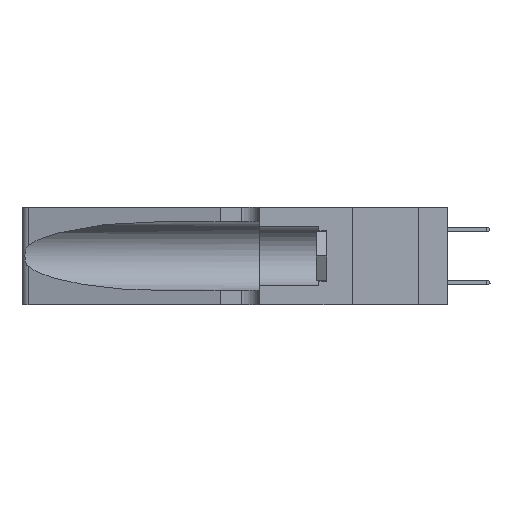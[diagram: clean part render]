
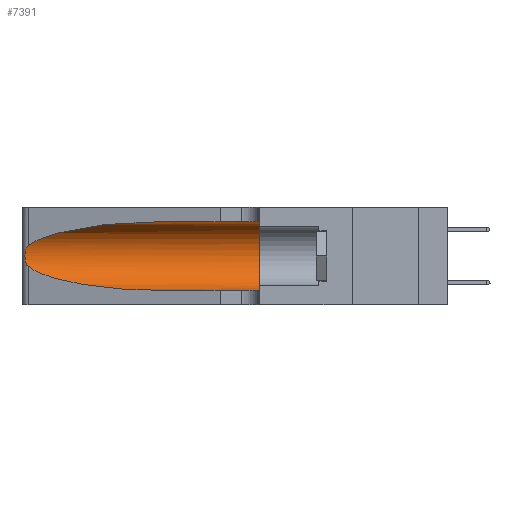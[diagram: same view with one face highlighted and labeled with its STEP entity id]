
A CAD part, left-side view. The second image highlights one B-rep face of the part: STEP entity #7391.
In plain terms, the highlighted cylindrical face has radius 3.308 mm (diameter 6.617 mm), a partial arc.
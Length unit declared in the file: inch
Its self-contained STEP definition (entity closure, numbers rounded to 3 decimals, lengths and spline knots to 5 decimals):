
#606 = CARTESIAN_POINT ( 'NONE',  ( 0.26017, 1.23833, 0.17102 ) ) ;
#2856 = EDGE_CURVE ( 'NONE', #10969, #3639, #28377, .T. ) ;
#3639 = VERTEX_POINT ( 'NONE', #48839 ) ;
#4372 = CARTESIAN_POINT ( 'NONE',  ( 0.25487, 1.22718, 0.22369 ) ) ;
#4533 = CARTESIAN_POINT ( 'NONE',  ( 0.25789, 1.23486, 0.15765 ) ) ;
#5224 = DIRECTION ( 'NONE',  ( 0., -1., 0. ) ) ;
#5656 = CARTESIAN_POINT ( 'NONE',  ( 0.1305, 1.61858, 0.05475 ) ) ;
#5905 = EDGE_CURVE ( 'NONE', #47473, #48548, #41609, .T. ) ;
#6003 = CARTESIAN_POINT ( 'NONE',  ( 0.25487, 1.22718, 0.14631 ) ) ;
#6124 = ORIENTED_EDGE ( 'NONE', *, *, #35734, .F. ) ;
#7391 = ADVANCED_FACE ( 'NONE', ( #47871 ), #16689, .F. ) ;
#8394 = CARTESIAN_POINT ( 'NONE',  ( 0.25555, 1.22993, 0.14849 ) ) ;
#8513 = EDGE_CURVE ( 'NONE', #26982, #40452, #19558, .T. ) ;
#10969 = VERTEX_POINT ( 'NONE', #30127 ) ;
#11135 = CARTESIAN_POINT ( 'NONE',  ( 0.2373, 1.15595, 0.08982 ) ) ;
#11461 = CARTESIAN_POINT ( 'NONE',  ( 0.18966, 0.96281, 0.05475 ) ) ;
#14625 = LINE ( 'NONE', #5656, #23511 ) ;
#15844 = CARTESIAN_POINT ( 'NONE',  ( 0.25787, 1.23484, 0.2124 ) ) ;
#16093 = ORIENTED_EDGE ( 'NONE', *, *, #2856, .T. ) ;
#16689 = CYLINDRICAL_SURFACE ( 'NONE', #29745, 0.13025 ) ;
#19558 =( BOUNDED_CURVE ( )  B_SPLINE_CURVE ( 3, ( #30328, #11135, #11461, #37866 ),
 .UNSPECIFIED., .F., .F. ) 
 B_SPLINE_CURVE_WITH_KNOTS ( ( 4, 4 ),
 ( 3.44316, 4.71239 ),
 .UNSPECIFIED. ) 
 CURVE ( )  GEOMETRIC_REPRESENTATION_ITEM ( )  RATIONAL_B_SPLINE_CURVE ( ( 1., 0.87, 0.87, 1. ) ) 
 REPRESENTATION_ITEM ( '' )  );
#19678 = CARTESIAN_POINT ( 'NONE',  ( 0.26018, 1.23835, 0.19895 ) ) ;
#20430 = CARTESIAN_POINT ( 'NONE',  ( 0.1305, 0.35, 0.185 ) ) ;
#22636 = CARTESIAN_POINT ( 'NONE',  ( 0.1305, 1.61858, 0.31525 ) ) ;
#23462 = CARTESIAN_POINT ( 'NONE',  ( 0.26075, 1.23896, 0.178 ) ) ;
#23511 = VECTOR ( 'NONE', #35915, 39.37008 ) ;
#24247 = DIRECTION ( 'NONE',  ( 0., 0., 1. ) ) ;
#24736 = B_SPLINE_CURVE_WITH_KNOTS ( 'NONE', 3,
 ( #4372, #42047, #38439, #15844, #42210, #19678, #45951, #23462, #606, #27323, #4533, #31049, #8394, #34835 ),
 .UNSPECIFIED., .F., .F.,
 ( 4, 2, 2, 2, 2, 2, 4 ),
 ( 0., 0.00027, 0.00053, 0.00107, 0.0016, 0.00187, 0.00214 ),
 .UNSPECIFIED. ) ;
#26568 = CARTESIAN_POINT ( 'NONE',  ( 0.18966, 0.96281, 0.31525 ) ) ;
#26982 = VERTEX_POINT ( 'NONE', #6003 ) ;
#27323 = CARTESIAN_POINT ( 'NONE',  ( 0.25856, 1.23593, 0.16098 ) ) ;
#27991 = CARTESIAN_POINT ( 'NONE',  ( 0.1305, 1.61858, 0.185 ) ) ;
#28377 =( BOUNDED_CURVE ( )  B_SPLINE_CURVE ( 3, ( #30321, #26568, #48971, #34089 ),
 .UNSPECIFIED., .F., .F. ) 
 B_SPLINE_CURVE_WITH_KNOTS ( ( 4, 4 ),
 ( 1.5708, 2.84003 ),
 .UNSPECIFIED. ) 
 CURVE ( )  GEOMETRIC_REPRESENTATION_ITEM ( )  RATIONAL_B_SPLINE_CURVE ( ( 1., 0.87, 0.87, 1. ) ) 
 REPRESENTATION_ITEM ( '' )  );
#29745 = AXIS2_PLACEMENT_3D ( 'NONE', #27991, #5224, #31721 ) ;
#30127 = CARTESIAN_POINT ( 'NONE',  ( 0.1305, 0.72297, 0.31525 ) ) ;
#30321 = CARTESIAN_POINT ( 'NONE',  ( 0.1305, 0.72297, 0.31525 ) ) ;
#30328 = CARTESIAN_POINT ( 'NONE',  ( 0.25487, 1.22718, 0.14631 ) ) ;
#30532 = CARTESIAN_POINT ( 'NONE',  ( 0.1305, 0.72297, 0.05475 ) ) ;
#30937 = AXIS2_PLACEMENT_3D ( 'NONE', #20430, #46700, #24247 ) ;
#31049 = CARTESIAN_POINT ( 'NONE',  ( 0.25639, 1.23186, 0.15144 ) ) ;
#31544 = ORIENTED_EDGE ( 'NONE', *, *, #5905, .F. ) ;
#31620 = EDGE_CURVE ( 'NONE', #3639, #26982, #24736, .T. ) ;
#31721 = DIRECTION ( 'NONE',  ( 0., 0., -1. ) ) ;
#32508 = EDGE_CURVE ( 'NONE', #40452, #48548, #14625, .T. ) ;
#34089 = CARTESIAN_POINT ( 'NONE',  ( 0.25487, 1.22718, 0.22369 ) ) ;
#34835 = CARTESIAN_POINT ( 'NONE',  ( 0.25487, 1.22718, 0.14631 ) ) ;
#35734 = EDGE_CURVE ( 'NONE', #10969, #47473, #41620, .T. ) ;
#35915 = DIRECTION ( 'NONE',  ( 0., -1., 0. ) ) ;
#36234 = ORIENTED_EDGE ( 'NONE', *, *, #32508, .T. ) ;
#37866 = CARTESIAN_POINT ( 'NONE',  ( 0.1305, 0.72297, 0.05475 ) ) ;
#38439 = CARTESIAN_POINT ( 'NONE',  ( 0.25639, 1.23184, 0.21858 ) ) ;
#38453 = EDGE_LOOP ( 'NONE', ( #16093, #40838, #41447, #36234, #31544, #6124 ) ) ;
#39949 = CARTESIAN_POINT ( 'NONE',  ( 0.1305, 0.35, 0.05475 ) ) ;
#40451 = VECTOR ( 'NONE', #45112, 39.37008 ) ;
#40452 = VERTEX_POINT ( 'NONE', #30532 ) ;
#40838 = ORIENTED_EDGE ( 'NONE', *, *, #31620, .T. ) ;
#41447 = ORIENTED_EDGE ( 'NONE', *, *, #8513, .T. ) ;
#41609 = CIRCLE ( 'NONE', #30937, 0.13025 ) ;
#41620 = LINE ( 'NONE', #22636, #40451 ) ;
#42047 = CARTESIAN_POINT ( 'NONE',  ( 0.25555, 1.22994, 0.2215 ) ) ;
#42210 = CARTESIAN_POINT ( 'NONE',  ( 0.25854, 1.2359, 0.20912 ) ) ;
#45101 = CARTESIAN_POINT ( 'NONE',  ( 0.1305, 0.35, 0.31525 ) ) ;
#45112 = DIRECTION ( 'NONE',  ( 0., -1., 0. ) ) ;
#45951 = CARTESIAN_POINT ( 'NONE',  ( 0.26075, 1.23896, 0.19203 ) ) ;
#46700 = DIRECTION ( 'NONE',  ( 0., 1., 0. ) ) ;
#47473 = VERTEX_POINT ( 'NONE', #45101 ) ;
#47871 = FACE_OUTER_BOUND ( 'NONE', #38453, .T. ) ;
#48548 = VERTEX_POINT ( 'NONE', #39949 ) ;
#48839 = CARTESIAN_POINT ( 'NONE',  ( 0.25487, 1.22718, 0.22369 ) ) ;
#48971 = CARTESIAN_POINT ( 'NONE',  ( 0.2373, 1.15595, 0.28018 ) ) ;
